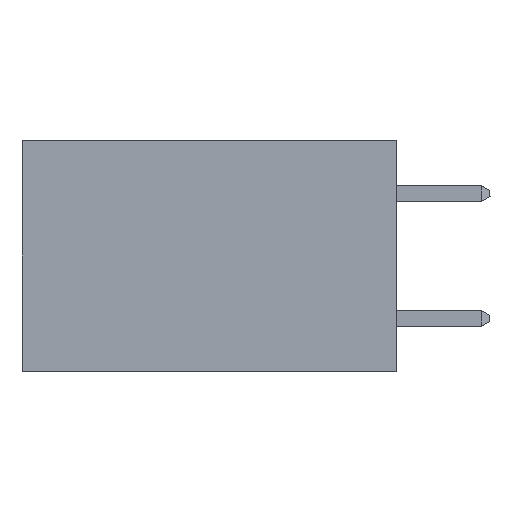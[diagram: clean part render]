
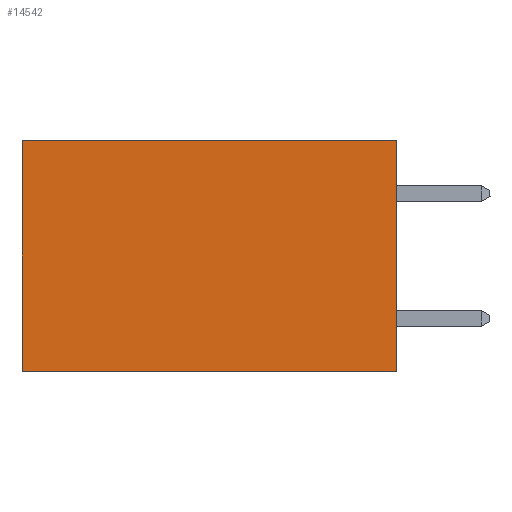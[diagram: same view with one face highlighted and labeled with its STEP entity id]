
A CAD part, left-side view. The second image highlights one B-rep face of the part: STEP entity #14542.
In plain terms, the highlighted planar face has unit normal (-1, 0, 0).
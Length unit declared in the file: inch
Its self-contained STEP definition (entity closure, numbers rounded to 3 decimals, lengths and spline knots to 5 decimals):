
#84 = ORIENTED_EDGE ( 'NONE', *, *, #2235, .T. ) ;
#681 = LINE ( 'NONE', #14803, #1662 ) ;
#1092 = ORIENTED_EDGE ( 'NONE', *, *, #12333, .F. ) ;
#1662 = VECTOR ( 'NONE', #5012, 39.37008 ) ;
#2235 = EDGE_CURVE ( 'NONE', #11195, #9949, #9181, .T. ) ;
#2278 = PLANE ( 'NONE',  #6564 ) ;
#2569 = VECTOR ( 'NONE', #11609, 39.37008 ) ;
#2663 = CARTESIAN_POINT ( 'NONE',  ( 0.298, 0., -0.37 ) ) ;
#3261 = ORIENTED_EDGE ( 'NONE', *, *, #3543, .T. ) ;
#3486 = ORIENTED_EDGE ( 'NONE', *, *, #14783, .F. ) ;
#3543 = EDGE_CURVE ( 'NONE', #15812, #11195, #15939, .T. ) ;
#3700 = CARTESIAN_POINT ( 'NONE',  ( 0.298, 0.6, 0. ) ) ;
#5012 = DIRECTION ( 'NONE',  ( 0., 0., -1. ) ) ;
#5957 = DIRECTION ( 'NONE',  ( 1., 0., 0. ) ) ;
#6051 = CARTESIAN_POINT ( 'NONE',  ( 0.298, 0., 0. ) ) ;
#6564 = AXIS2_PLACEMENT_3D ( 'NONE', #9535, #5957, #12051 ) ;
#7041 = CARTESIAN_POINT ( 'NONE',  ( 0.298, 0., 0. ) ) ;
#7277 = LINE ( 'NONE', #11219, #12925 ) ;
#7445 = VERTEX_POINT ( 'NONE', #2663 ) ;
#8641 = DIRECTION ( 'NONE',  ( 0., 1., 0. ) ) ;
#9157 = CARTESIAN_POINT ( 'NONE',  ( 0.298, 0.6, -0.37 ) ) ;
#9181 = LINE ( 'NONE', #15311, #2569 ) ;
#9535 = CARTESIAN_POINT ( 'NONE',  ( 0.298, 0., 0. ) ) ;
#9949 = VERTEX_POINT ( 'NONE', #9157 ) ;
#11081 = VECTOR ( 'NONE', #13450, 39.37008 ) ;
#11195 = VERTEX_POINT ( 'NONE', #3700 ) ;
#11219 = CARTESIAN_POINT ( 'NONE',  ( 0.298, 0., -0.37 ) ) ;
#11609 = DIRECTION ( 'NONE',  ( 0., 0., -1. ) ) ;
#12051 = DIRECTION ( 'NONE',  ( 0., 0., -1. ) ) ;
#12333 = EDGE_CURVE ( 'NONE', #15812, #7445, #681, .T. ) ;
#12925 = VECTOR ( 'NONE', #8641, 39.37008 ) ;
#13450 = DIRECTION ( 'NONE',  ( 0., 1., 0. ) ) ;
#14341 = EDGE_LOOP ( 'NONE', ( #84, #3486, #1092, #3261 ) ) ;
#14542 = ADVANCED_FACE ( 'NONE', ( #16050 ), #2278, .F. ) ;
#14783 = EDGE_CURVE ( 'NONE', #7445, #9949, #7277, .T. ) ;
#14803 = CARTESIAN_POINT ( 'NONE',  ( 0.298, 0., 0. ) ) ;
#15311 = CARTESIAN_POINT ( 'NONE',  ( 0.298, 0.6, 0. ) ) ;
#15812 = VERTEX_POINT ( 'NONE', #7041 ) ;
#15939 = LINE ( 'NONE', #6051, #11081 ) ;
#16050 = FACE_OUTER_BOUND ( 'NONE', #14341, .T. ) ;
